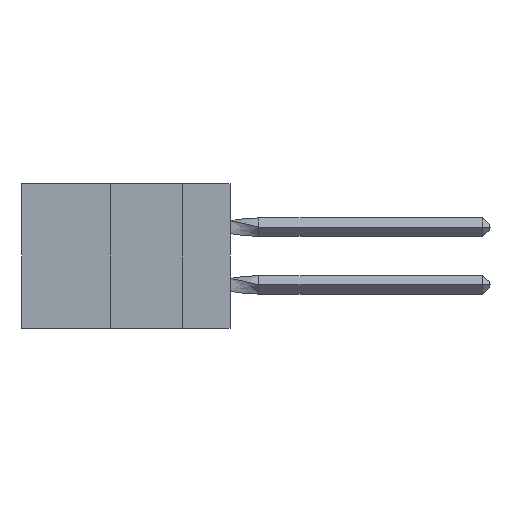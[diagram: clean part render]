
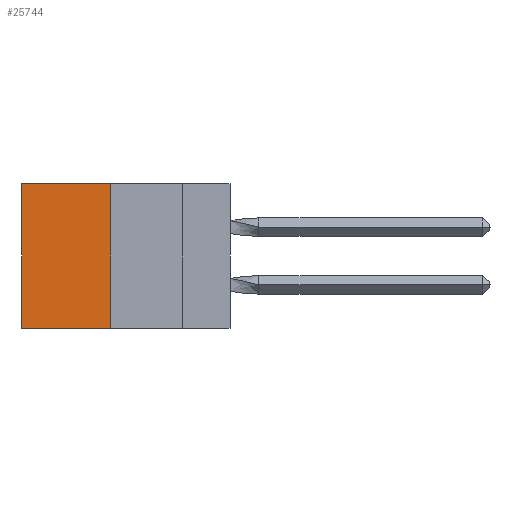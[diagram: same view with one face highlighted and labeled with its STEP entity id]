
A CAD part, left-side view. The second image highlights one B-rep face of the part: STEP entity #25744.
In plain terms, the highlighted planar face has unit normal (-1, 0, 0).
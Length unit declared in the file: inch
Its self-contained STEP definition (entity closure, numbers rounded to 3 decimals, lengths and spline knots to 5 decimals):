
#112 = CARTESIAN_POINT ( 'NONE',  ( 0.305, 0.413, -0.5 ) ) ;
#1410 = VECTOR ( 'NONE', #21573, 39.37008 ) ;
#2250 = VECTOR ( 'NONE', #32603, 39.37008 ) ;
#2483 = CARTESIAN_POINT ( 'NONE',  ( 0.305, 0.413, 0. ) ) ;
#3201 = LINE ( 'NONE', #7421, #1410 ) ;
#5184 = CARTESIAN_POINT ( 'NONE',  ( 0.305, 0.413, -0.5 ) ) ;
#6189 = FACE_OUTER_BOUND ( 'NONE', #17659, .T. ) ;
#6405 = ORIENTED_EDGE ( 'NONE', *, *, #34956, .F. ) ;
#6530 = VECTOR ( 'NONE', #26748, 39.37008 ) ;
#6698 = CARTESIAN_POINT ( 'NONE',  ( 0.305, 0.413, -0.5 ) ) ;
#7421 = CARTESIAN_POINT ( 'NONE',  ( 0.305, 0.72, -0.5 ) ) ;
#8674 = VECTOR ( 'NONE', #26431, 39.37008 ) ;
#10791 = ORIENTED_EDGE ( 'NONE', *, *, #11027, .F. ) ;
#11027 = EDGE_CURVE ( 'NONE', #12918, #35321, #13602, .T. ) ;
#12918 = VERTEX_POINT ( 'NONE', #2483 ) ;
#13602 = LINE ( 'NONE', #112, #8674 ) ;
#13613 = CARTESIAN_POINT ( 'NONE',  ( 0.305, 0.413, -0.5 ) ) ;
#16744 = CARTESIAN_POINT ( 'NONE',  ( 0.305, 0.72, -0.5 ) ) ;
#16951 = PLANE ( 'NONE',  #25709 ) ;
#17472 = CARTESIAN_POINT ( 'NONE',  ( 0.305, 0.72, 0. ) ) ;
#17659 = EDGE_LOOP ( 'NONE', ( #29133, #6405, #10791, #32956 ) ) ;
#21573 = DIRECTION ( 'NONE',  ( 0., 0., -1. ) ) ;
#21825 = EDGE_CURVE ( 'NONE', #12918, #30399, #36682, .T. ) ;
#24646 = LINE ( 'NONE', #6698, #2250 ) ;
#25709 = AXIS2_PLACEMENT_3D ( 'NONE', #5184, #31181, #28148 ) ;
#25744 = ADVANCED_FACE ( 'NONE', ( #6189 ), #16951, .F. ) ;
#26431 = DIRECTION ( 'NONE',  ( 0., 0., -1. ) ) ;
#26521 = CARTESIAN_POINT ( 'NONE',  ( 0.305, 0.413, 0. ) ) ;
#26748 = DIRECTION ( 'NONE',  ( 0., 1., 0. ) ) ;
#28148 = DIRECTION ( 'NONE',  ( 0., 0., -1. ) ) ;
#29133 = ORIENTED_EDGE ( 'NONE', *, *, #30786, .T. ) ;
#30399 = VERTEX_POINT ( 'NONE', #17472 ) ;
#30786 = EDGE_CURVE ( 'NONE', #30399, #36450, #3201, .T. ) ;
#31181 = DIRECTION ( 'NONE',  ( 1., 0., 0. ) ) ;
#32603 = DIRECTION ( 'NONE',  ( 0., 1., 0. ) ) ;
#32956 = ORIENTED_EDGE ( 'NONE', *, *, #21825, .T. ) ;
#34956 = EDGE_CURVE ( 'NONE', #35321, #36450, #24646, .T. ) ;
#35321 = VERTEX_POINT ( 'NONE', #13613 ) ;
#36450 = VERTEX_POINT ( 'NONE', #16744 ) ;
#36682 = LINE ( 'NONE', #26521, #6530 ) ;
